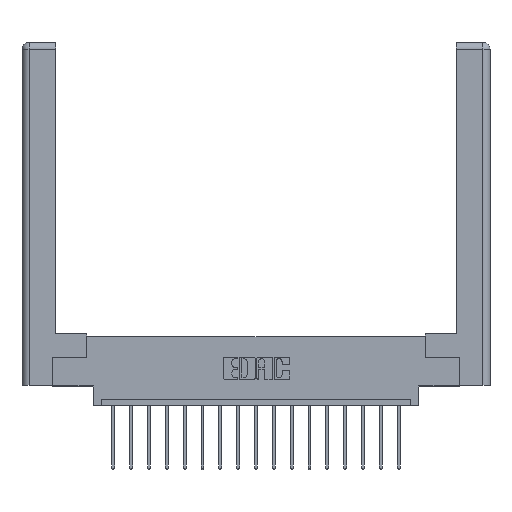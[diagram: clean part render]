
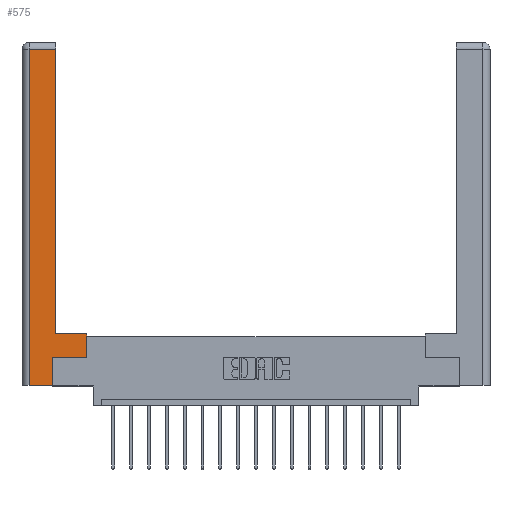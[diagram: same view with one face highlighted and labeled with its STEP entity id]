
A CAD part, top view. The second image highlights one B-rep face of the part: STEP entity #575.
In plain terms, the highlighted planar face has unit normal (0, 0, 1).
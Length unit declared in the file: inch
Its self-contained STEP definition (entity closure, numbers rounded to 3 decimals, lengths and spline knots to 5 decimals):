
#166 = CARTESIAN_POINT ( 'NONE',  ( 0.295, 0.45, 0. ) ) ;
#236 = DIRECTION ( 'NONE',  ( -1., 0., 0. ) ) ;
#531 = VECTOR ( 'NONE', #16178, 39.37008 ) ;
#551 = LINE ( 'NONE', #3558, #10017 ) ;
#575 = ADVANCED_FACE ( 'NONE', ( #5278 ), #11635, .F. ) ;
#718 = VERTEX_POINT ( 'NONE', #16101 ) ;
#1020 = CARTESIAN_POINT ( 'NONE',  ( 0.295, 0.45, 0. ) ) ;
#1234 = ORIENTED_EDGE ( 'NONE', *, *, #12493, .T. ) ;
#1245 = CARTESIAN_POINT ( 'NONE',  ( 0.565, 0.45, 0. ) ) ;
#1314 = CARTESIAN_POINT ( 'NONE',  ( 0.265, 0., 0. ) ) ;
#1373 = AXIS2_PLACEMENT_3D ( 'NONE', #14306, #10052, #11381 ) ;
#1628 = VECTOR ( 'NONE', #13170, 39.37008 ) ;
#2275 = DIRECTION ( 'NONE',  ( 1., 0., 0. ) ) ;
#3444 = VECTOR ( 'NONE', #16800, 39.37008 ) ;
#3558 = CARTESIAN_POINT ( 'NONE',  ( 0.565, 0.245, 0. ) ) ;
#3757 = ORIENTED_EDGE ( 'NONE', *, *, #17379, .T. ) ;
#3813 = VECTOR ( 'NONE', #2275, 39.37008 ) ;
#4029 = ORIENTED_EDGE ( 'NONE', *, *, #12006, .T. ) ;
#4196 = VERTEX_POINT ( 'NONE', #7210 ) ;
#4489 = CARTESIAN_POINT ( 'NONE',  ( 0.0615, 2.94, 0. ) ) ;
#4512 = VECTOR ( 'NONE', #8446, 39.37008 ) ;
#4540 = EDGE_LOOP ( 'NONE', ( #1234, #16898, #4029, #18680, #6945, #3757, #10322, #5646 ) ) ;
#4980 = LINE ( 'NONE', #1245, #4512 ) ;
#5224 = EDGE_CURVE ( 'NONE', #12997, #10114, #10569, .T. ) ;
#5278 = FACE_OUTER_BOUND ( 'NONE', #4540, .T. ) ;
#5488 = EDGE_CURVE ( 'NONE', #4196, #13699, #5826, .T. ) ;
#5646 = ORIENTED_EDGE ( 'NONE', *, *, #5224, .T. ) ;
#5737 = VERTEX_POINT ( 'NONE', #6178 ) ;
#5826 = LINE ( 'NONE', #8161, #3813 ) ;
#6178 = CARTESIAN_POINT ( 'NONE',  ( 0.0615, 2.94, 0. ) ) ;
#6461 = DIRECTION ( 'NONE',  ( 1., 0., 0. ) ) ;
#6680 = EDGE_CURVE ( 'NONE', #16758, #5737, #11425, .T. ) ;
#6945 = ORIENTED_EDGE ( 'NONE', *, *, #8051, .T. ) ;
#7210 = CARTESIAN_POINT ( 'NONE',  ( 0.0615, 0., 0. ) ) ;
#7440 = CARTESIAN_POINT ( 'NONE',  ( 0.565, 0.45, 0. ) ) ;
#7619 = VECTOR ( 'NONE', #236, 39.37008 ) ;
#8051 = EDGE_CURVE ( 'NONE', #13699, #718, #12285, .T. ) ;
#8161 = CARTESIAN_POINT ( 'NONE',  ( 0.265, 0., 0. ) ) ;
#8225 = CARTESIAN_POINT ( 'NONE',  ( 0.265, 0.245, 0. ) ) ;
#8446 = DIRECTION ( 'NONE',  ( 0., 1., 0. ) ) ;
#9315 = LINE ( 'NONE', #18619, #1628 ) ;
#9998 = LINE ( 'NONE', #17750, #531 ) ;
#10017 = VECTOR ( 'NONE', #6461, 39.37008 ) ;
#10052 = DIRECTION ( 'NONE',  ( 0., 0., -1. ) ) ;
#10114 = VERTEX_POINT ( 'NONE', #1020 ) ;
#10322 = ORIENTED_EDGE ( 'NONE', *, *, #13686, .T. ) ;
#10563 = DIRECTION ( 'NONE',  ( -1., 0., 0. ) ) ;
#10569 = LINE ( 'NONE', #166, #7619 ) ;
#11012 = VERTEX_POINT ( 'NONE', #15455 ) ;
#11381 = DIRECTION ( 'NONE',  ( -1., 0., 0. ) ) ;
#11425 = LINE ( 'NONE', #4489, #14379 ) ;
#11635 = PLANE ( 'NONE',  #1373 ) ;
#12006 = EDGE_CURVE ( 'NONE', #5737, #4196, #9998, .T. ) ;
#12285 = LINE ( 'NONE', #8225, #3444 ) ;
#12493 = EDGE_CURVE ( 'NONE', #10114, #16758, #9315, .T. ) ;
#12997 = VERTEX_POINT ( 'NONE', #7440 ) ;
#13170 = DIRECTION ( 'NONE',  ( 0., 1., 0. ) ) ;
#13686 = EDGE_CURVE ( 'NONE', #11012, #12997, #4980, .T. ) ;
#13699 = VERTEX_POINT ( 'NONE', #1314 ) ;
#14306 = CARTESIAN_POINT ( 'NONE',  ( 0., 0., 0. ) ) ;
#14379 = VECTOR ( 'NONE', #10563, 39.37008 ) ;
#15455 = CARTESIAN_POINT ( 'NONE',  ( 0.565, 0.245, 0. ) ) ;
#16101 = CARTESIAN_POINT ( 'NONE',  ( 0.265, 0.245, 0. ) ) ;
#16178 = DIRECTION ( 'NONE',  ( 0., -1., 0. ) ) ;
#16206 = CARTESIAN_POINT ( 'NONE',  ( 0.295, 2.94, 0. ) ) ;
#16758 = VERTEX_POINT ( 'NONE', #16206 ) ;
#16800 = DIRECTION ( 'NONE',  ( 0., 1., 0. ) ) ;
#16898 = ORIENTED_EDGE ( 'NONE', *, *, #6680, .T. ) ;
#17379 = EDGE_CURVE ( 'NONE', #718, #11012, #551, .T. ) ;
#17750 = CARTESIAN_POINT ( 'NONE',  ( 0.0615, 0., 0. ) ) ;
#18619 = CARTESIAN_POINT ( 'NONE',  ( 0.295, 3., 0. ) ) ;
#18680 = ORIENTED_EDGE ( 'NONE', *, *, #5488, .T. ) ;
